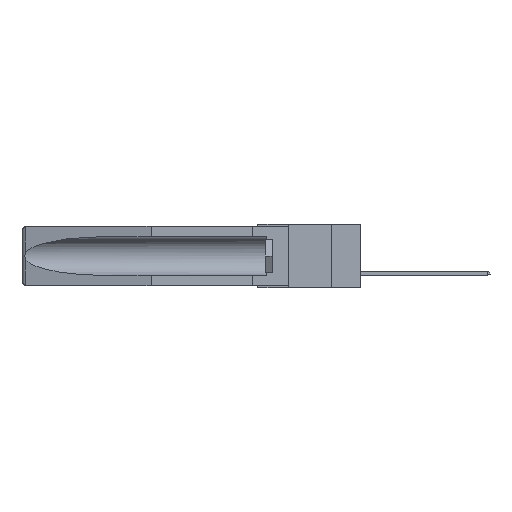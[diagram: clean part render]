
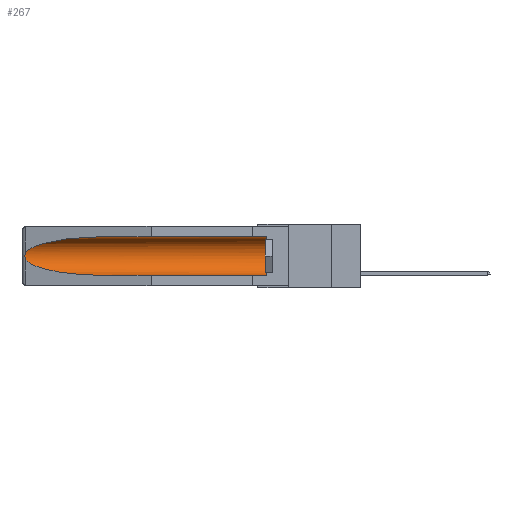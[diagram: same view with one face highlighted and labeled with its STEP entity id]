
A CAD part, left-side view. The second image highlights one B-rep face of the part: STEP entity #267.
In plain terms, the highlighted cylindrical face has radius 2.857 mm (diameter 5.715 mm), a partial arc.
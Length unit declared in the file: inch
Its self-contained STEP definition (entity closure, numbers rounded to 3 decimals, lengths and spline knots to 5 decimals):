
#267 = ADVANCED_FACE ( 'NONE', ( #8428 ), #13030, .F. ) ;
#1115 = DIRECTION ( 'NONE',  ( 0., -1., 0. ) ) ;
#1819 =( BOUNDED_CURVE ( )  B_SPLINE_CURVE ( 3, ( #2689, #4443, #11108, #20127 ),
 .UNSPECIFIED., .F., .T. ) 
 B_SPLINE_CURVE_WITH_KNOTS ( ( 4, 4 ),
 ( 0.1948, 1.5708 ),
 .UNSPECIFIED. ) 
 CURVE ( )  GEOMETRIC_REPRESENTATION_ITEM ( )  RATIONAL_B_SPLINE_CURVE ( ( 1., 0.848, 0.848, 1. ) ) 
 REPRESENTATION_ITEM ( '' )  );
#2103 =( BOUNDED_CURVE ( )  B_SPLINE_CURVE ( 3, ( #10759, #7366, #12440, #17633 ),
 .UNSPECIFIED., .F., .F. ) 
 B_SPLINE_CURVE_WITH_KNOTS ( ( 4, 4 ),
 ( 4.71239, 6.08839 ),
 .UNSPECIFIED. ) 
 CURVE ( )  GEOMETRIC_REPRESENTATION_ITEM ( )  RATIONAL_B_SPLINE_CURVE ( ( 1., 0.848, 0.848, 1. ) ) 
 REPRESENTATION_ITEM ( '' )  );
#2294 = EDGE_CURVE ( 'NONE', #18124, #19988, #21689, .T. ) ;
#2414 = ORIENTED_EDGE ( 'NONE', *, *, #2294, .T. ) ;
#2503 = VECTOR ( 'NONE', #20316, 39.37008 ) ;
#2689 = CARTESIAN_POINT ( 'NONE',  ( 0.26537, 1.52718, -0.19328 ) ) ;
#2865 = EDGE_LOOP ( 'NONE', ( #19960, #3457, #7569, #20056, #19495, #2414 ) ) ;
#2878 = CARTESIAN_POINT ( 'NONE',  ( 0.2675, 1.53308, -0.16763 ) ) ;
#3200 = VERTEX_POINT ( 'NONE', #20639 ) ;
#3457 = ORIENTED_EDGE ( 'NONE', *, *, #10263, .T. ) ;
#3730 = CARTESIAN_POINT ( 'NONE',  ( 0.155, -0.30754, -0.059 ) ) ;
#4443 = CARTESIAN_POINT ( 'NONE',  ( 0.25451, 1.48313, -0.24835 ) ) ;
#4662 = CARTESIAN_POINT ( 'NONE',  ( 0.26655, 1.53094, -0.18657 ) ) ;
#4897 = CARTESIAN_POINT ( 'NONE',  ( 0.155, 1.07973, -0.059 ) ) ;
#5256 = EDGE_CURVE ( 'NONE', #5322, #3200, #8770, .T. ) ;
#5270 = DIRECTION ( 'NONE',  ( 0., 1., 0. ) ) ;
#5322 = VERTEX_POINT ( 'NONE', #13662 ) ;
#5979 = DIRECTION ( 'NONE',  ( 0., 0., 1. ) ) ;
#6388 = CARTESIAN_POINT ( 'NONE',  ( 0.26597, 1.5296, -0.19026 ) ) ;
#7240 = CARTESIAN_POINT ( 'NONE',  ( 0.26537, 1.52718, -0.19328 ) ) ;
#7366 = CARTESIAN_POINT ( 'NONE',  ( 0.21114, 1.30732, -0.059 ) ) ;
#7569 = ORIENTED_EDGE ( 'NONE', *, *, #11176, .T. ) ;
#8143 = CARTESIAN_POINT ( 'NONE',  ( 0.2673, 1.53269, -0.17917 ) ) ;
#8216 = CARTESIAN_POINT ( 'NONE',  ( 0.26537, 1.52718, -0.19328 ) ) ;
#8428 = FACE_OUTER_BOUND ( 'NONE', #2865, .T. ) ;
#8737 = VERTEX_POINT ( 'NONE', #7240 ) ;
#8770 = LINE ( 'NONE', #15287, #2503 ) ;
#9201 = DIRECTION ( 'NONE',  ( 0., 0., 1. ) ) ;
#9859 = VERTEX_POINT ( 'NONE', #21288 ) ;
#10263 = EDGE_CURVE ( 'NONE', #9859, #8737, #18975, .T. ) ;
#10759 = CARTESIAN_POINT ( 'NONE',  ( 0.155, 1.07973, -0.059 ) ) ;
#10863 = CARTESIAN_POINT ( 'NONE',  ( 0.155, -0.30754, -0.1715 ) ) ;
#11108 = CARTESIAN_POINT ( 'NONE',  ( 0.21114, 1.30732, -0.284 ) ) ;
#11176 = EDGE_CURVE ( 'NONE', #8737, #3200, #1819, .T. ) ;
#11490 = CARTESIAN_POINT ( 'NONE',  ( 0.155, 0.126, -0.1715 ) ) ;
#11522 = CARTESIAN_POINT ( 'NONE',  ( 0.26654, 1.53092, -0.15636 ) ) ;
#12440 = CARTESIAN_POINT ( 'NONE',  ( 0.25451, 1.48313, -0.09465 ) ) ;
#12925 = VECTOR ( 'NONE', #5270, 39.37008 ) ;
#13030 = CYLINDRICAL_SURFACE ( 'NONE', #21818, 0.1125 ) ;
#13370 = CARTESIAN_POINT ( 'NONE',  ( 0.2673, 1.5327, -0.16383 ) ) ;
#13662 = CARTESIAN_POINT ( 'NONE',  ( 0.155, 0.126, -0.284 ) ) ;
#15050 = CARTESIAN_POINT ( 'NONE',  ( 0.2675, 1.53308, -0.17534 ) ) ;
#15287 = CARTESIAN_POINT ( 'NONE',  ( 0.155, -0.30754, -0.284 ) ) ;
#15362 = CARTESIAN_POINT ( 'NONE',  ( 0.26537, 1.52718, -0.14972 ) ) ;
#15596 = CARTESIAN_POINT ( 'NONE',  ( 0.155, 0.126, -0.059 ) ) ;
#17158 = CIRCLE ( 'NONE', #19972, 0.1125 ) ;
#17633 = CARTESIAN_POINT ( 'NONE',  ( 0.26537, 1.52718, -0.14972 ) ) ;
#18124 = VERTEX_POINT ( 'NONE', #15596 ) ;
#18975 = B_SPLINE_CURVE_WITH_KNOTS ( 'NONE', 3,
 ( #15362, #22010, #11522, #13370, #2878, #15050, #8143, #4662, #6388, #8216 ),
 .UNSPECIFIED., .F., .F.,
 ( 4, 2, 2, 2, 4 ),
 ( 0., 0.00029, 0.00058, 0.00087, 0.00117 ),
 .UNSPECIFIED. ) ;
#19495 = ORIENTED_EDGE ( 'NONE', *, *, #20756, .T. ) ;
#19960 = ORIENTED_EDGE ( 'NONE', *, *, #20290, .T. ) ;
#19972 = AXIS2_PLACEMENT_3D ( 'NONE', #11490, #1115, #5979 ) ;
#19988 = VERTEX_POINT ( 'NONE', #4897 ) ;
#20056 = ORIENTED_EDGE ( 'NONE', *, *, #5256, .F. ) ;
#20127 = CARTESIAN_POINT ( 'NONE',  ( 0.155, 1.07973, -0.284 ) ) ;
#20290 = EDGE_CURVE ( 'NONE', #19988, #9859, #2103, .T. ) ;
#20316 = DIRECTION ( 'NONE',  ( 0., 1., 0. ) ) ;
#20639 = CARTESIAN_POINT ( 'NONE',  ( 0.155, 1.07973, -0.284 ) ) ;
#20756 = EDGE_CURVE ( 'NONE', #5322, #18124, #17158, .T. ) ;
#21288 = CARTESIAN_POINT ( 'NONE',  ( 0.26537, 1.52718, -0.14972 ) ) ;
#21569 = DIRECTION ( 'NONE',  ( 0., 1., 0. ) ) ;
#21689 = LINE ( 'NONE', #3730, #12925 ) ;
#21818 = AXIS2_PLACEMENT_3D ( 'NONE', #10863, #21569, #9201 ) ;
#22010 = CARTESIAN_POINT ( 'NONE',  ( 0.26597, 1.52961, -0.15275 ) ) ;
